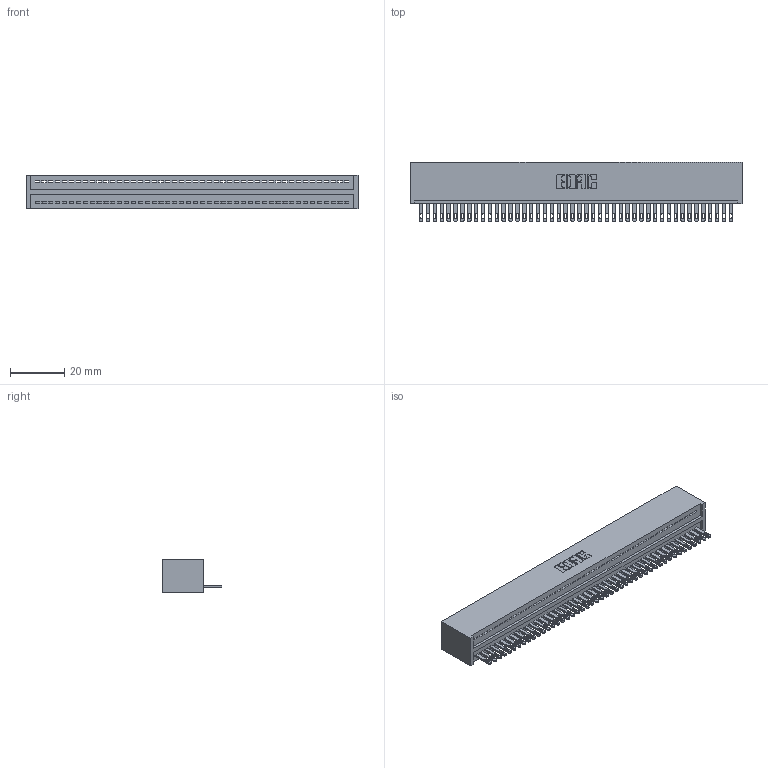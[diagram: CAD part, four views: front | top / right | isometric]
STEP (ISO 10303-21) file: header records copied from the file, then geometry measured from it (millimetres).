
FILE_DESCRIPTION (( 'STEP AP203' ), '1' );
FILE_NAME ('325-046-500-101.STEP', '2020-02-24T22:44:20', ( '' ), ( '' ), 'SwSTEP 2.0', 'SolidWorks 2016', '' );
FILE_SCHEMA (( 'CONFIG_CONTROL_DESIGN' ));
Length unit declared in the file: inch
Products named in the file (3): 325-046-500-101; 325-292-001_325-293-100; 325 Part_Lugless
Assembly tree (47 placements, depth 2):
  325-046-500-101
    325 Part_Lugless
    325-292-001_325-293-100  x46
Bounding box: 122.48 x 21.84 x 12.45 mm (x, y, z)
Volume: 16180.4 mm3; surface area: 18343 mm2
Topology: 47 solids, 47 shells, 2590 faces, 8015 edges, 5342 vertices
Faces by surface type: plane 1722, cylinder 868
Entity records: 27257 total; most frequent: CARTESIAN_POINT 4708, ORIENTED_EDGE 4690, DIRECTION 3957, EDGE_CURVE 2345, LINE 2221, VECTOR 2221, VERTEX_POINT 1562, AXIS2_PLACEMENT_3D 868
